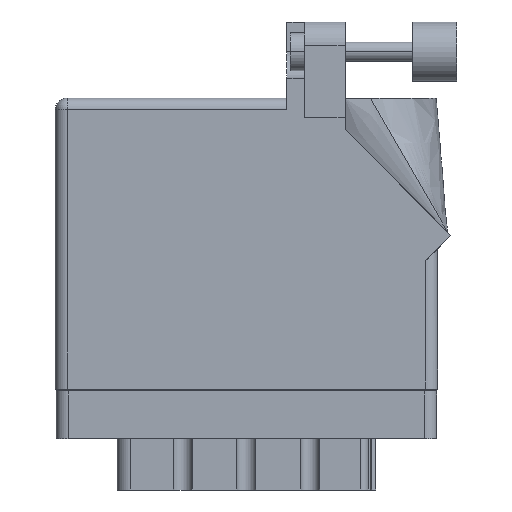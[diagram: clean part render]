
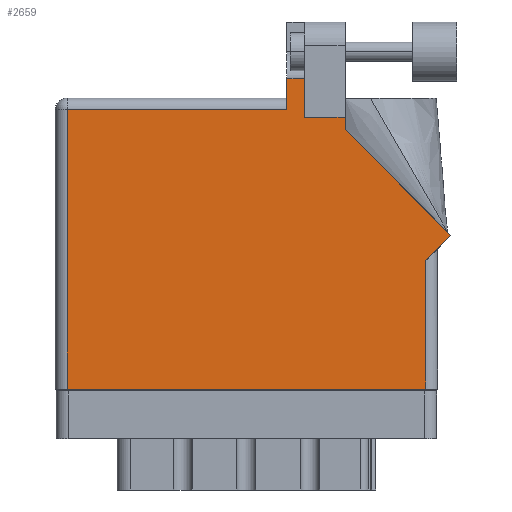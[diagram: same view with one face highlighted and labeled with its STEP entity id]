
A CAD part, front view. The second image highlights one B-rep face of the part: STEP entity #2659.
In plain terms, the highlighted face is planar.
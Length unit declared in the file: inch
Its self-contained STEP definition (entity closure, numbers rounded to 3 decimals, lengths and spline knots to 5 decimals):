
#250 = VECTOR ( 'NONE', #24631, 39.37008 ) ;
#418 = CARTESIAN_POINT ( 'NONE',  ( 2.08071, 0.80771, 0. ) ) ;
#750 = EDGE_CURVE ( 'NONE', #9005, #12539, #16278, .T. ) ;
#1575 = VERTEX_POINT ( 'NONE', #21217 ) ;
#2184 = CARTESIAN_POINT ( 'NONE',  ( 0., 1.468, 0. ) ) ;
#2659 = ADVANCED_FACE ( 'NONE', ( #24677 ), #28173, .F. ) ;
#2786 = CARTESIAN_POINT ( 'NONE',  ( 0.062, 0., 0. ) ) ;
#3257 = CARTESIAN_POINT ( 'NONE',  ( 0., 1.53, 0. ) ) ;
#3266 = EDGE_CURVE ( 'NONE', #1575, #29927, #6306, .T. ) ;
#3572 = CARTESIAN_POINT ( 'NONE',  ( 1.217, 1.468, 0. ) ) ;
#3881 = EDGE_CURVE ( 'NONE', #19967, #1575, #13537, .T. ) ;
#4297 = CARTESIAN_POINT ( 'NONE',  ( 1.311, 1.6315, 0. ) ) ;
#5010 = EDGE_CURVE ( 'NONE', #20316, #18383, #15859, .T. ) ;
#5180 = EDGE_CURVE ( 'NONE', #14973, #20316, #13818, .T. ) ;
#5621 = AXIS2_PLACEMENT_3D ( 'NONE', #3257, #16046, #26351 ) ;
#6306 = LINE ( 'NONE', #15317, #23320 ) ;
#6601 = VECTOR ( 'NONE', #14932, 39.37008 ) ;
#8853 = EDGE_CURVE ( 'NONE', #13535, #14973, #23289, .T. ) ;
#8992 = VECTOR ( 'NONE', #10643, 39.37008 ) ;
#9005 = VERTEX_POINT ( 'NONE', #3572 ) ;
#9934 = VERTEX_POINT ( 'NONE', #19723 ) ;
#10643 = DIRECTION ( 'NONE',  ( -0.707, 0.707, 0. ) ) ;
#10742 = CARTESIAN_POINT ( 'NONE',  ( 0.062, 1.468, 0. ) ) ;
#11478 = LINE ( 'NONE', #17684, #6601 ) ;
#11520 = ORIENTED_EDGE ( 'NONE', *, *, #20526, .T. ) ;
#11682 = DIRECTION ( 'NONE',  ( -1., 0., 0. ) ) ;
#11833 = VECTOR ( 'NONE', #30077, 39.37008 ) ;
#12243 = ORIENTED_EDGE ( 'NONE', *, *, #5180, .T. ) ;
#12539 = VERTEX_POINT ( 'NONE', #10742 ) ;
#12565 = DIRECTION ( 'NONE',  ( -1., 0., 0. ) ) ;
#12945 = CARTESIAN_POINT ( 'NONE',  ( 0.062, 0., 0. ) ) ;
#13139 = VERTEX_POINT ( 'NONE', #12945 ) ;
#13296 = ORIENTED_EDGE ( 'NONE', *, *, #8853, .T. ) ;
#13535 = VERTEX_POINT ( 'NONE', #14751 ) ;
#13537 = LINE ( 'NONE', #15051, #27324 ) ;
#13697 = ORIENTED_EDGE ( 'NONE', *, *, #5010, .T. ) ;
#13818 = LINE ( 'NONE', #31917, #11833 ) ;
#14164 = DIRECTION ( 'NONE',  ( 1., 0., 0. ) ) ;
#14355 = ORIENTED_EDGE ( 'NONE', *, *, #15758, .T. ) ;
#14751 = CARTESIAN_POINT ( 'NONE',  ( 1.948, 0., 0. ) ) ;
#14932 = DIRECTION ( 'NONE',  ( 0., 1., 0. ) ) ;
#14973 = VERTEX_POINT ( 'NONE', #15650 ) ;
#15051 = CARTESIAN_POINT ( 'NONE',  ( 1.524, 1.43, 0. ) ) ;
#15317 = CARTESIAN_POINT ( 'NONE',  ( 1.311, 1.43, 0. ) ) ;
#15650 = CARTESIAN_POINT ( 'NONE',  ( 1.948, 0.675, 0. ) ) ;
#15758 = EDGE_CURVE ( 'NONE', #29927, #9934, #24753, .T. ) ;
#15859 = LINE ( 'NONE', #418, #8992 ) ;
#16046 = DIRECTION ( 'NONE',  ( 0., 0., -1. ) ) ;
#16278 = LINE ( 'NONE', #2184, #23965 ) ;
#16289 = VECTOR ( 'NONE', #26448, 39.37008 ) ;
#17684 = CARTESIAN_POINT ( 'NONE',  ( 1.524, 1.36442, 0. ) ) ;
#17790 = CARTESIAN_POINT ( 'NONE',  ( 2.08071, 0.80771, 0. ) ) ;
#18383 = VERTEX_POINT ( 'NONE', #26812 ) ;
#19561 = VECTOR ( 'NONE', #21227, 39.37008 ) ;
#19582 = CARTESIAN_POINT ( 'NONE',  ( 1.64177, 1.6315, 0. ) ) ;
#19723 = CARTESIAN_POINT ( 'NONE',  ( 1.217, 1.6315, 0. ) ) ;
#19967 = VERTEX_POINT ( 'NONE', #28841 ) ;
#20313 = EDGE_CURVE ( 'NONE', #18383, #19967, #11478, .T. ) ;
#20316 = VERTEX_POINT ( 'NONE', #17790 ) ;
#20526 = EDGE_CURVE ( 'NONE', #12539, #13139, #27248, .T. ) ;
#21217 = CARTESIAN_POINT ( 'NONE',  ( 1.311, 1.43, 0. ) ) ;
#21227 = DIRECTION ( 'NONE',  ( 0., -1., 0. ) ) ;
#22674 = EDGE_CURVE ( 'NONE', #13139, #13535, #31950, .T. ) ;
#23289 = LINE ( 'NONE', #28921, #16289 ) ;
#23320 = VECTOR ( 'NONE', #33018, 39.37008 ) ;
#23669 = EDGE_LOOP ( 'NONE', ( #31781, #14355, #24299, #26590, #11520, #23758, #13296, #12243, #13697, #32710, #32277 ) ) ;
#23707 = EDGE_CURVE ( 'NONE', #9934, #9005, #25372, .T. ) ;
#23758 = ORIENTED_EDGE ( 'NONE', *, *, #22674, .T. ) ;
#23965 = VECTOR ( 'NONE', #25178, 39.37008 ) ;
#24231 = VECTOR ( 'NONE', #14164, 39.37008 ) ;
#24299 = ORIENTED_EDGE ( 'NONE', *, *, #23707, .T. ) ;
#24631 = DIRECTION ( 'NONE',  ( 0., -1., 0. ) ) ;
#24677 = FACE_OUTER_BOUND ( 'NONE', #23669, .T. ) ;
#24753 = LINE ( 'NONE', #19582, #30008 ) ;
#25178 = DIRECTION ( 'NONE',  ( -1., 0., 0. ) ) ;
#25372 = LINE ( 'NONE', #32244, #250 ) ;
#26351 = DIRECTION ( 'NONE',  ( -1., 0., 0. ) ) ;
#26448 = DIRECTION ( 'NONE',  ( 0., 1., 0. ) ) ;
#26590 = ORIENTED_EDGE ( 'NONE', *, *, #750, .T. ) ;
#26812 = CARTESIAN_POINT ( 'NONE',  ( 1.524, 1.36442, 0. ) ) ;
#26845 = CARTESIAN_POINT ( 'NONE',  ( 0., 0., 0. ) ) ;
#27248 = LINE ( 'NONE', #2786, #19561 ) ;
#27324 = VECTOR ( 'NONE', #12565, 39.37008 ) ;
#28173 = PLANE ( 'NONE',  #5621 ) ;
#28841 = CARTESIAN_POINT ( 'NONE',  ( 1.524, 1.43, 0. ) ) ;
#28921 = CARTESIAN_POINT ( 'NONE',  ( 1.948, 0.737, 0. ) ) ;
#29927 = VERTEX_POINT ( 'NONE', #4297 ) ;
#30008 = VECTOR ( 'NONE', #11682, 39.37008 ) ;
#30077 = DIRECTION ( 'NONE',  ( 0.707, 0.707, 0. ) ) ;
#31781 = ORIENTED_EDGE ( 'NONE', *, *, #3266, .T. ) ;
#31917 = CARTESIAN_POINT ( 'NONE',  ( 2.01, 0.737, 0. ) ) ;
#31950 = LINE ( 'NONE', #26845, #24231 ) ;
#32244 = CARTESIAN_POINT ( 'NONE',  ( 1.217, 1.53, 0. ) ) ;
#32277 = ORIENTED_EDGE ( 'NONE', *, *, #3881, .T. ) ;
#32710 = ORIENTED_EDGE ( 'NONE', *, *, #20313, .T. ) ;
#33018 = DIRECTION ( 'NONE',  ( 0., 1., 0. ) ) ;
